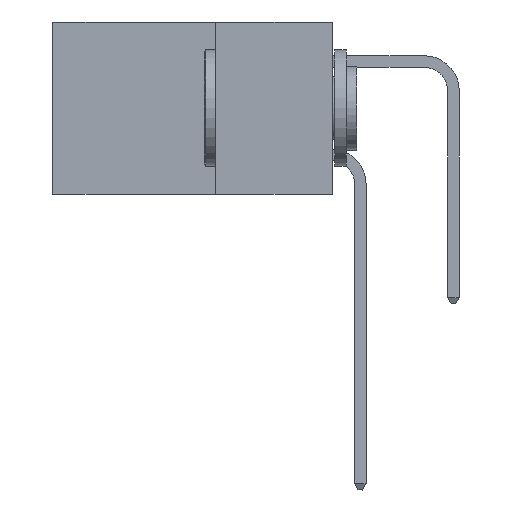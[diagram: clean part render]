
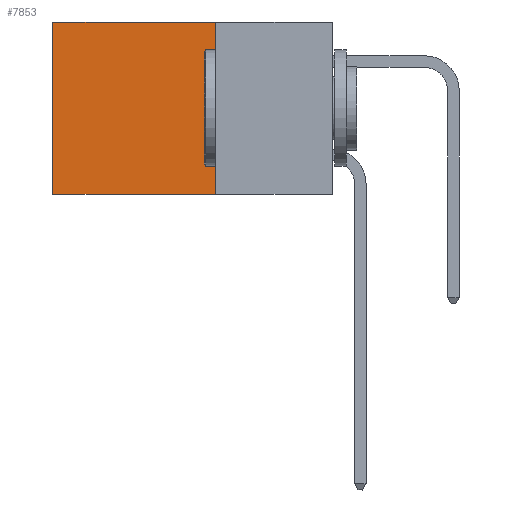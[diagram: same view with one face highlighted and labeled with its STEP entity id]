
A CAD part, left-side view. The second image highlights one B-rep face of the part: STEP entity #7853.
In plain terms, the highlighted planar face has unit normal (-1, 0, 0).
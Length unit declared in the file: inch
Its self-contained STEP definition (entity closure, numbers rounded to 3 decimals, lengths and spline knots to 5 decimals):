
#442 = CARTESIAN_POINT ( 'NONE',  ( 0.2615, 0.6, 0. ) ) ;
#1051 = AXIS2_PLACEMENT_3D ( 'NONE', #4525, #2112, #3586 ) ;
#1154 = EDGE_CURVE ( 'NONE', #13371, #8143, #12533, .T. ) ;
#1474 = ORIENTED_EDGE ( 'NONE', *, *, #14320, .F. ) ;
#2021 = ORIENTED_EDGE ( 'NONE', *, *, #1154, .T. ) ;
#2112 = DIRECTION ( 'NONE',  ( 1., 0., 0. ) ) ;
#2176 = DIRECTION ( 'NONE',  ( 0., 0., -1. ) ) ;
#2418 = PLANE ( 'NONE',  #1051 ) ;
#2551 = VERTEX_POINT ( 'NONE', #13752 ) ;
#2578 = EDGE_LOOP ( 'NONE', ( #2021, #1474, #13952, #9459 ) ) ;
#2925 = DIRECTION ( 'NONE',  ( 0., 1., 0. ) ) ;
#3292 = DIRECTION ( 'NONE',  ( 0., 1., 0. ) ) ;
#3586 = DIRECTION ( 'NONE',  ( 0., 0., -1. ) ) ;
#4216 = DIRECTION ( 'NONE',  ( 0., 0., -1. ) ) ;
#4525 = CARTESIAN_POINT ( 'NONE',  ( 0.2615, 0.25, -0.37 ) ) ;
#4937 = CARTESIAN_POINT ( 'NONE',  ( 0.2615, 0.25, 0. ) ) ;
#5697 = EDGE_CURVE ( 'NONE', #7612, #13371, #13841, .T. ) ;
#6299 = VECTOR ( 'NONE', #2925, 39.37008 ) ;
#7612 = VERTEX_POINT ( 'NONE', #4937 ) ;
#7853 = ADVANCED_FACE ( 'NONE', ( #13087 ), #2418, .F. ) ;
#8143 = VERTEX_POINT ( 'NONE', #8875 ) ;
#8875 = CARTESIAN_POINT ( 'NONE',  ( 0.2615, 0.6, -0.37 ) ) ;
#9459 = ORIENTED_EDGE ( 'NONE', *, *, #5697, .T. ) ;
#9505 = LINE ( 'NONE', #9583, #14504 ) ;
#9583 = CARTESIAN_POINT ( 'NONE',  ( 0.2615, 0.25, -0.37 ) ) ;
#10279 = EDGE_CURVE ( 'NONE', #7612, #2551, #9505, .T. ) ;
#10286 = CARTESIAN_POINT ( 'NONE',  ( 0.2615, 0.25, 0. ) ) ;
#10496 = LINE ( 'NONE', #11757, #12439 ) ;
#10500 = VECTOR ( 'NONE', #4216, 39.37008 ) ;
#11757 = CARTESIAN_POINT ( 'NONE',  ( 0.2615, 0.25, -0.37 ) ) ;
#12439 = VECTOR ( 'NONE', #3292, 39.37008 ) ;
#12533 = LINE ( 'NONE', #15141, #10500 ) ;
#13087 = FACE_OUTER_BOUND ( 'NONE', #2578, .T. ) ;
#13371 = VERTEX_POINT ( 'NONE', #442 ) ;
#13752 = CARTESIAN_POINT ( 'NONE',  ( 0.2615, 0.25, -0.37 ) ) ;
#13841 = LINE ( 'NONE', #10286, #6299 ) ;
#13952 = ORIENTED_EDGE ( 'NONE', *, *, #10279, .F. ) ;
#14320 = EDGE_CURVE ( 'NONE', #2551, #8143, #10496, .T. ) ;
#14504 = VECTOR ( 'NONE', #2176, 39.37008 ) ;
#15141 = CARTESIAN_POINT ( 'NONE',  ( 0.2615, 0.6, -0.37 ) ) ;
